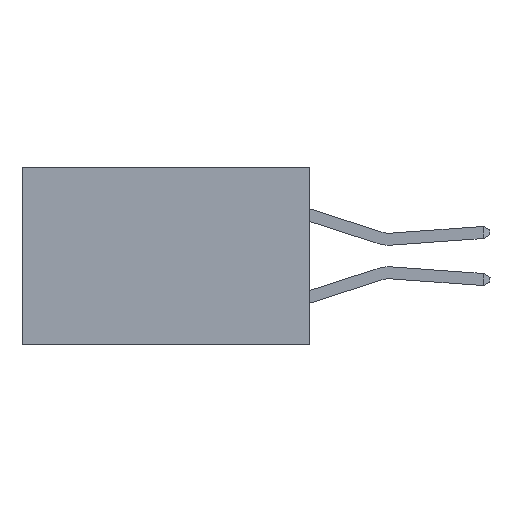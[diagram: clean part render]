
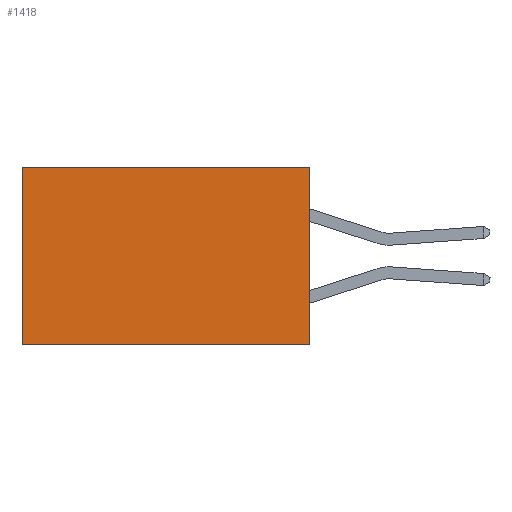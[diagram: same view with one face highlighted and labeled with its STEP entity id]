
A CAD part, left-side view. The second image highlights one B-rep face of the part: STEP entity #1418.
In plain terms, the highlighted planar face has unit normal (-1, 0, 0).
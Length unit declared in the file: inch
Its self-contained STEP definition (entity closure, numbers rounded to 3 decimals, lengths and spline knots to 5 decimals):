
#205 = CARTESIAN_POINT ( 'NONE',  ( 0.298, 0.6, 0. ) ) ;
#833 = ORIENTED_EDGE ( 'NONE', *, *, #8136, .T. ) ;
#925 = EDGE_CURVE ( 'NONE', #7500, #11729, #23954, .T. ) ;
#1054 = DIRECTION ( 'NONE',  ( 0., 0., -1. ) ) ;
#1418 = ADVANCED_FACE ( 'NONE', ( #3734 ), #13373, .F. ) ;
#2276 = EDGE_CURVE ( 'NONE', #11729, #7070, #19663, .T. ) ;
#2717 = LINE ( 'NONE', #10316, #21836 ) ;
#3734 = FACE_OUTER_BOUND ( 'NONE', #19116, .T. ) ;
#4304 = VECTOR ( 'NONE', #12313, 39.37008 ) ;
#4941 = CARTESIAN_POINT ( 'NONE',  ( 0.298, 0., 0. ) ) ;
#5012 = VERTEX_POINT ( 'NONE', #205 ) ;
#5578 = ORIENTED_EDGE ( 'NONE', *, *, #17452, .T. ) ;
#7070 = VERTEX_POINT ( 'NONE', #14709 ) ;
#7440 = VECTOR ( 'NONE', #1054, 39.37008 ) ;
#7500 = VERTEX_POINT ( 'NONE', #10745 ) ;
#8136 = EDGE_CURVE ( 'NONE', #5012, #7070, #22109, .T. ) ;
#10316 = CARTESIAN_POINT ( 'NONE',  ( 0.298, 0., 0. ) ) ;
#10745 = CARTESIAN_POINT ( 'NONE',  ( 0.298, 0., 0. ) ) ;
#11729 = VERTEX_POINT ( 'NONE', #16018 ) ;
#12313 = DIRECTION ( 'NONE',  ( 0., 1., 0. ) ) ;
#12318 = CARTESIAN_POINT ( 'NONE',  ( 0.298, 0.6, 0. ) ) ;
#12458 = DIRECTION ( 'NONE',  ( 0., 0., -1. ) ) ;
#13078 = DIRECTION ( 'NONE',  ( 1., 0., 0. ) ) ;
#13373 = PLANE ( 'NONE',  #20292 ) ;
#13614 = ORIENTED_EDGE ( 'NONE', *, *, #925, .F. ) ;
#13726 = VECTOR ( 'NONE', #12458, 39.37008 ) ;
#13747 = CARTESIAN_POINT ( 'NONE',  ( 0.298, 0., 0. ) ) ;
#14709 = CARTESIAN_POINT ( 'NONE',  ( 0.298, 0.6, -0.37 ) ) ;
#16018 = CARTESIAN_POINT ( 'NONE',  ( 0.298, 0., -0.37 ) ) ;
#17306 = CARTESIAN_POINT ( 'NONE',  ( 0.298, 0., -0.37 ) ) ;
#17452 = EDGE_CURVE ( 'NONE', #7500, #5012, #2717, .T. ) ;
#19116 = EDGE_LOOP ( 'NONE', ( #833, #19626, #13614, #5578 ) ) ;
#19463 = DIRECTION ( 'NONE',  ( 0., 1., 0. ) ) ;
#19626 = ORIENTED_EDGE ( 'NONE', *, *, #2276, .F. ) ;
#19663 = LINE ( 'NONE', #17306, #4304 ) ;
#20292 = AXIS2_PLACEMENT_3D ( 'NONE', #13747, #13078, #23339 ) ;
#21836 = VECTOR ( 'NONE', #19463, 39.37008 ) ;
#22109 = LINE ( 'NONE', #12318, #7440 ) ;
#23339 = DIRECTION ( 'NONE',  ( 0., 0., -1. ) ) ;
#23954 = LINE ( 'NONE', #4941, #13726 ) ;
